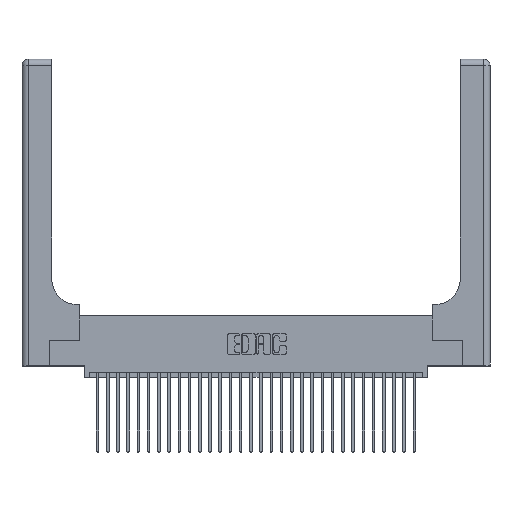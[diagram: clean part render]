
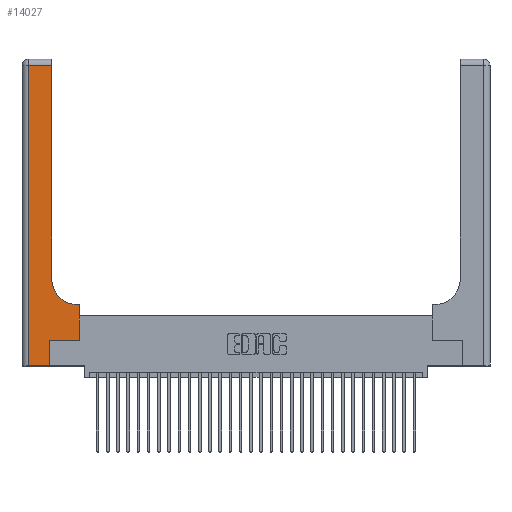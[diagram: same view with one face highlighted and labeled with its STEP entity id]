
A CAD part, top view. The second image highlights one B-rep face of the part: STEP entity #14027.
In plain terms, the highlighted planar face has unit normal (0, 0, 1).
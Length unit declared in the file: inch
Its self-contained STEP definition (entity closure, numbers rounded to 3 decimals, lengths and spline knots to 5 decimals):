
#214 = VERTEX_POINT ( 'NONE', #19308 ) ;
#227 = DIRECTION ( 'NONE',  ( 0., 1., 0. ) ) ;
#1842 = CARTESIAN_POINT ( 'NONE',  ( 0.06, 0., 0.37 ) ) ;
#3340 = CARTESIAN_POINT ( 'NONE',  ( 0.2915, 0.85, 0.37 ) ) ;
#3420 = PLANE ( 'NONE',  #26468 ) ;
#3525 = EDGE_CURVE ( 'NONE', #10411, #7933, #15321, .T. ) ;
#3578 = ORIENTED_EDGE ( 'NONE', *, *, #17322, .T. ) ;
#3637 = DIRECTION ( 'NONE',  ( -1., 0., 0. ) ) ;
#3645 = ORIENTED_EDGE ( 'NONE', *, *, #9538, .T. ) ;
#3744 = VECTOR ( 'NONE', #18708, 39.37008 ) ;
#3774 = EDGE_CURVE ( 'NONE', #30171, #15073, #27980, .T. ) ;
#4058 = DIRECTION ( 'NONE',  ( 1., 0., 0. ) ) ;
#4697 = LINE ( 'NONE', #31255, #11606 ) ;
#6219 = DIRECTION ( 'NONE',  ( 0., 1., 0. ) ) ;
#6356 = CARTESIAN_POINT ( 'NONE',  ( 0.2915, 3., 0.37 ) ) ;
#6383 = EDGE_CURVE ( 'NONE', #28577, #10411, #19890, .T. ) ;
#7029 = VERTEX_POINT ( 'NONE', #28149 ) ;
#7413 = CARTESIAN_POINT ( 'NONE',  ( 0.5585, 0.25, 0.37 ) ) ;
#7518 = CARTESIAN_POINT ( 'NONE',  ( 0.2915, 0.6, 0.37 ) ) ;
#7933 = VERTEX_POINT ( 'NONE', #31552 ) ;
#8021 = CARTESIAN_POINT ( 'NONE',  ( 0.06, 2.94, 0.37 ) ) ;
#8036 = AXIS2_PLACEMENT_3D ( 'NONE', #8619, #8721, #4058 ) ;
#8041 = ORIENTED_EDGE ( 'NONE', *, *, #10942, .T. ) ;
#8260 = EDGE_LOOP ( 'NONE', ( #8041, #24152, #18611, #18646, #3578, #24225, #10246, #9946, #3645 ) ) ;
#8619 = CARTESIAN_POINT ( 'NONE',  ( 0.5415, 0.85, 0.37 ) ) ;
#8721 = DIRECTION ( 'NONE',  ( 0., 0., -1. ) ) ;
#9538 = EDGE_CURVE ( 'NONE', #15073, #31546, #14716, .T. ) ;
#9679 = EDGE_CURVE ( 'NONE', #7029, #214, #13545, .T. ) ;
#9897 = VECTOR ( 'NONE', #25002, 39.37008 ) ;
#9946 = ORIENTED_EDGE ( 'NONE', *, *, #3774, .T. ) ;
#10246 = ORIENTED_EDGE ( 'NONE', *, *, #24224, .T. ) ;
#10411 = VERTEX_POINT ( 'NONE', #1842 ) ;
#10843 = DIRECTION ( 'NONE',  ( 0., 0., -1. ) ) ;
#10942 = EDGE_CURVE ( 'NONE', #31546, #28633, #23467, .T. ) ;
#11132 = DIRECTION ( 'NONE',  ( 0., 1., 0. ) ) ;
#11606 = VECTOR ( 'NONE', #6219, 39.37008 ) ;
#12169 = LINE ( 'NONE', #31309, #22173 ) ;
#12332 = VECTOR ( 'NONE', #11132, 39.37008 ) ;
#12644 = CARTESIAN_POINT ( 'NONE',  ( 0.06, 3., 0.37 ) ) ;
#13545 = LINE ( 'NONE', #23570, #25842 ) ;
#13573 = CARTESIAN_POINT ( 'NONE',  ( 0., 0., 0.37 ) ) ;
#14027 = ADVANCED_FACE ( 'NONE', ( #30320 ), #3420, .F. ) ;
#14716 = CIRCLE ( 'NONE', #8036, 0.25 ) ;
#15073 = VERTEX_POINT ( 'NONE', #25376 ) ;
#15321 = LINE ( 'NONE', #13573, #3744 ) ;
#16647 = VECTOR ( 'NONE', #227, 39.37008 ) ;
#16831 = VECTOR ( 'NONE', #17029, 39.37008 ) ;
#17029 = DIRECTION ( 'NONE',  ( -1., 0., 0. ) ) ;
#17322 = EDGE_CURVE ( 'NONE', #7933, #7029, #4697, .T. ) ;
#18611 = ORIENTED_EDGE ( 'NONE', *, *, #6383, .T. ) ;
#18646 = ORIENTED_EDGE ( 'NONE', *, *, #3525, .T. ) ;
#18708 = DIRECTION ( 'NONE',  ( 1., 0., 0. ) ) ;
#19308 = CARTESIAN_POINT ( 'NONE',  ( 0.5585, 0.25, 0.37 ) ) ;
#19876 = CARTESIAN_POINT ( 'NONE',  ( 0.5585, 0.6, 0.37 ) ) ;
#19890 = LINE ( 'NONE', #12644, #9897 ) ;
#21078 = DIRECTION ( 'NONE',  ( 1., 0., 0. ) ) ;
#22015 = EDGE_CURVE ( 'NONE', #28633, #28577, #12169, .T. ) ;
#22173 = VECTOR ( 'NONE', #26301, 39.37008 ) ;
#23089 = CARTESIAN_POINT ( 'NONE',  ( 0., 3., 0.37 ) ) ;
#23467 = LINE ( 'NONE', #6356, #12332 ) ;
#23570 = CARTESIAN_POINT ( 'NONE',  ( 0.269, 0.25, 0.37 ) ) ;
#24152 = ORIENTED_EDGE ( 'NONE', *, *, #22015, .T. ) ;
#24224 = EDGE_CURVE ( 'NONE', #214, #30171, #28935, .T. ) ;
#24225 = ORIENTED_EDGE ( 'NONE', *, *, #9679, .T. ) ;
#25002 = DIRECTION ( 'NONE',  ( 0., -1., 0. ) ) ;
#25234 = CARTESIAN_POINT ( 'NONE',  ( 0.2915, 2.94, 0.37 ) ) ;
#25376 = CARTESIAN_POINT ( 'NONE',  ( 0.5415, 0.6, 0.37 ) ) ;
#25842 = VECTOR ( 'NONE', #21078, 39.37008 ) ;
#26301 = DIRECTION ( 'NONE',  ( -1., 0., 0. ) ) ;
#26468 = AXIS2_PLACEMENT_3D ( 'NONE', #23089, #10843, #3637 ) ;
#27980 = LINE ( 'NONE', #7518, #16831 ) ;
#28149 = CARTESIAN_POINT ( 'NONE',  ( 0.269, 0.25, 0.37 ) ) ;
#28577 = VERTEX_POINT ( 'NONE', #8021 ) ;
#28633 = VERTEX_POINT ( 'NONE', #25234 ) ;
#28935 = LINE ( 'NONE', #7413, #16647 ) ;
#30171 = VERTEX_POINT ( 'NONE', #19876 ) ;
#30320 = FACE_OUTER_BOUND ( 'NONE', #8260, .T. ) ;
#31255 = CARTESIAN_POINT ( 'NONE',  ( 0.269, 0., 0.37 ) ) ;
#31309 = CARTESIAN_POINT ( 'NONE',  ( 0., 2.94, 0.37 ) ) ;
#31546 = VERTEX_POINT ( 'NONE', #3340 ) ;
#31552 = CARTESIAN_POINT ( 'NONE',  ( 0.269, 0., 0.37 ) ) ;
